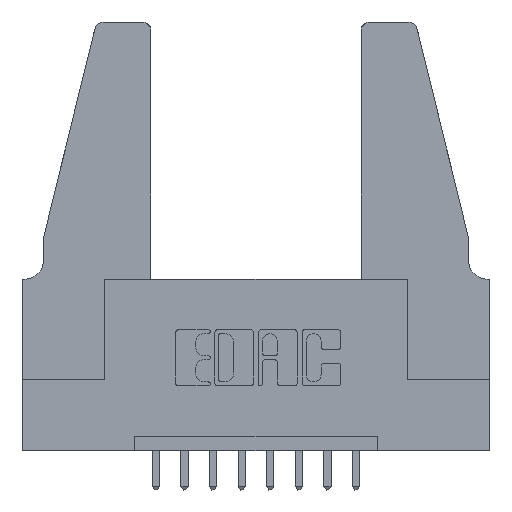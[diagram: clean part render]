
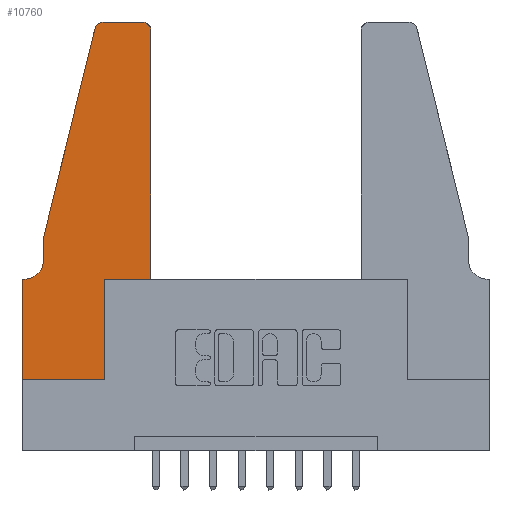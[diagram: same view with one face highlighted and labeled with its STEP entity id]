
A CAD part, top view. The second image highlights one B-rep face of the part: STEP entity #10760.
In plain terms, the highlighted planar face has unit normal (0, 0, 1).
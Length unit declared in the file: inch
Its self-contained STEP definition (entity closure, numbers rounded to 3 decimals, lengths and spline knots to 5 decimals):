
#9 = CARTESIAN_POINT ( 'NONE',  ( 0., 0.35, 0.37 ) ) ;
#29 = AXIS2_PLACEMENT_3D ( 'NONE', #9, #6821, #977 ) ;
#51 = ORIENTED_EDGE ( 'NONE', *, *, #4607, .T. ) ;
#342 = ORIENTED_EDGE ( 'NONE', *, *, #5918, .T. ) ;
#507 = VERTEX_POINT ( 'NONE', #11353 ) ;
#553 = DIRECTION ( 'NONE',  ( 0., -1., 0. ) ) ;
#571 = VECTOR ( 'NONE', #3005, 39.37008 ) ;
#877 = LINE ( 'NONE', #9490, #2388 ) ;
#940 = ORIENTED_EDGE ( 'NONE', *, *, #4984, .T. ) ;
#977 = DIRECTION ( 'NONE',  ( 1., 0., 0. ) ) ;
#985 = DIRECTION ( 'NONE',  ( -1., 0., 0. ) ) ;
#1038 = LINE ( 'NONE', #6354, #9707 ) ;
#1223 = VERTEX_POINT ( 'NONE', #7634 ) ;
#1245 = VERTEX_POINT ( 'NONE', #7879 ) ;
#1325 = VERTEX_POINT ( 'NONE', #9859 ) ;
#1500 = CARTESIAN_POINT ( 'NONE',  ( 0., 0.35, 0.37 ) ) ;
#1552 = CARTESIAN_POINT ( 'NONE',  ( 0., 0., 0.37 ) ) ;
#1948 = DIRECTION ( 'NONE',  ( 0., 0., 1. ) ) ;
#2105 = CARTESIAN_POINT ( 'NONE',  ( 0.0755, 0.5, 0.37 ) ) ;
#2178 = EDGE_CURVE ( 'NONE', #4876, #12113, #877, .T. ) ;
#2276 = LINE ( 'NONE', #6950, #5089 ) ;
#2388 = VECTOR ( 'NONE', #6645, 39.37008 ) ;
#2587 = CARTESIAN_POINT ( 'NONE',  ( 0.0755, 0.5, 0.37 ) ) ;
#2669 = ORIENTED_EDGE ( 'NONE', *, *, #11542, .T. ) ;
#3005 = DIRECTION ( 'NONE',  ( 0., 1., 0. ) ) ;
#3397 = CARTESIAN_POINT ( 'NONE',  ( 0.2865, 0., 0.37 ) ) ;
#3514 = EDGE_CURVE ( 'NONE', #1325, #11162, #4635, .T. ) ;
#3616 = CARTESIAN_POINT ( 'NONE',  ( 0.25487, 1.22718, 0.37 ) ) ;
#3918 = CARTESIAN_POINT ( 'NONE',  ( 0.4505, 0.35, 0.37 ) ) ;
#4117 = ORIENTED_EDGE ( 'NONE', *, *, #11129, .T. ) ;
#4183 = CARTESIAN_POINT ( 'NONE',  ( 0.0755, 0.42, 0.37 ) ) ;
#4236 = DIRECTION ( 'NONE',  ( -1., 0., 0. ) ) ;
#4283 = VECTOR ( 'NONE', #4236, 39.37008 ) ;
#4607 = EDGE_CURVE ( 'NONE', #7946, #507, #10639, .T. ) ;
#4635 = LINE ( 'NONE', #1552, #12669 ) ;
#4818 = PLANE ( 'NONE',  #29 ) ;
#4876 = VERTEX_POINT ( 'NONE', #3918 ) ;
#4931 = DIRECTION ( 'NONE',  ( 1., 0., 0. ) ) ;
#4984 = EDGE_CURVE ( 'NONE', #6380, #4876, #1038, .T. ) ;
#5089 = VECTOR ( 'NONE', #9927, 39.37008 ) ;
#5247 = VERTEX_POINT ( 'NONE', #2105 ) ;
#5677 = DIRECTION ( 'NONE',  ( 1., 0., 0. ) ) ;
#5882 = AXIS2_PLACEMENT_3D ( 'NONE', #9718, #9678, #12691 ) ;
#5918 = EDGE_CURVE ( 'NONE', #1245, #12586, #12764, .T. ) ;
#5923 = CARTESIAN_POINT ( 'NONE',  ( 0.0055, 0.42, 0.37 ) ) ;
#6045 = CARTESIAN_POINT ( 'NONE',  ( 0.2865, 0.35, 0.37 ) ) ;
#6167 = VECTOR ( 'NONE', #553, 39.37008 ) ;
#6354 = CARTESIAN_POINT ( 'NONE',  ( 0.4505, 0.35, 0.37 ) ) ;
#6380 = VERTEX_POINT ( 'NONE', #6488 ) ;
#6448 = AXIS2_PLACEMENT_3D ( 'NONE', #5923, #6925, #985 ) ;
#6488 = CARTESIAN_POINT ( 'NONE',  ( 0.2865, 0.35, 0.37 ) ) ;
#6645 = DIRECTION ( 'NONE',  ( 0., 1., 0. ) ) ;
#6821 = DIRECTION ( 'NONE',  ( 0., 0., 1. ) ) ;
#6925 = DIRECTION ( 'NONE',  ( 0., 0., -1. ) ) ;
#6950 = CARTESIAN_POINT ( 'NONE',  ( 0.0755, 0.35, 0.37 ) ) ;
#7523 = ORIENTED_EDGE ( 'NONE', *, *, #9766, .T. ) ;
#7634 = CARTESIAN_POINT ( 'NONE',  ( 0.4205, 1.25, 0.37 ) ) ;
#7635 = ORIENTED_EDGE ( 'NONE', *, *, #3514, .T. ) ;
#7644 = EDGE_LOOP ( 'NONE', ( #2669, #342, #12574, #8592, #51, #10507, #4117, #7635, #7523, #940, #10047, #9013 ) ) ;
#7724 = LINE ( 'NONE', #12223, #12016 ) ;
#7848 = LINE ( 'NONE', #9208, #4283 ) ;
#7879 = CARTESIAN_POINT ( 'NONE',  ( 0.284, 1.25, 0.37 ) ) ;
#7922 = CARTESIAN_POINT ( 'NONE',  ( 0.4505, 1.22, 0.37 ) ) ;
#7926 = VECTOR ( 'NONE', #11912, 39.37008 ) ;
#7946 = VERTEX_POINT ( 'NONE', #4183 ) ;
#8294 = DIRECTION ( 'NONE',  ( 0., -1., 0. ) ) ;
#8571 = EDGE_CURVE ( 'NONE', #12586, #5247, #12215, .T. ) ;
#8592 = ORIENTED_EDGE ( 'NONE', *, *, #10491, .T. ) ;
#9009 = CARTESIAN_POINT ( 'NONE',  ( 0.4205, 1.22, 0.37 ) ) ;
#9013 = ORIENTED_EDGE ( 'NONE', *, *, #11661, .T. ) ;
#9208 = CARTESIAN_POINT ( 'NONE',  ( 0.2605, 1.25, 0.37 ) ) ;
#9490 = CARTESIAN_POINT ( 'NONE',  ( 0.4505, 0.35, 0.37 ) ) ;
#9678 = DIRECTION ( 'NONE',  ( 0., 0., 1. ) ) ;
#9707 = VECTOR ( 'NONE', #11383, 39.37008 ) ;
#9718 = CARTESIAN_POINT ( 'NONE',  ( 0.284, 1.22, 0.37 ) ) ;
#9766 = EDGE_CURVE ( 'NONE', #11162, #6380, #10155, .T. ) ;
#9859 = CARTESIAN_POINT ( 'NONE',  ( 0., 0., 0.37 ) ) ;
#9927 = DIRECTION ( 'NONE',  ( -1., 0., 0. ) ) ;
#10047 = ORIENTED_EDGE ( 'NONE', *, *, #2178, .T. ) ;
#10109 = AXIS2_PLACEMENT_3D ( 'NONE', #9009, #1948, #4931 ) ;
#10155 = LINE ( 'NONE', #6045, #571 ) ;
#10390 = CARTESIAN_POINT ( 'NONE',  ( 0.0755, 0.5, 0.37 ) ) ;
#10491 = EDGE_CURVE ( 'NONE', #5247, #7946, #11578, .T. ) ;
#10507 = ORIENTED_EDGE ( 'NONE', *, *, #10699, .T. ) ;
#10639 = CIRCLE ( 'NONE', #6448, 0.07 ) ;
#10699 = EDGE_CURVE ( 'NONE', #507, #12460, #2276, .T. ) ;
#10760 = ADVANCED_FACE ( 'NONE', ( #11737 ), #4818, .T. ) ;
#11129 = EDGE_CURVE ( 'NONE', #12460, #1325, #7724, .T. ) ;
#11162 = VERTEX_POINT ( 'NONE', #3397 ) ;
#11353 = CARTESIAN_POINT ( 'NONE',  ( 0.0055, 0.35, 0.37 ) ) ;
#11383 = DIRECTION ( 'NONE',  ( 1., 0., 0. ) ) ;
#11542 = EDGE_CURVE ( 'NONE', #1223, #1245, #7848, .T. ) ;
#11578 = LINE ( 'NONE', #10390, #6167 ) ;
#11661 = EDGE_CURVE ( 'NONE', #12113, #1223, #12468, .T. ) ;
#11737 = FACE_OUTER_BOUND ( 'NONE', #7644, .T. ) ;
#11912 = DIRECTION ( 'NONE',  ( -0.239, -0.971, 0. ) ) ;
#12016 = VECTOR ( 'NONE', #8294, 39.37008 ) ;
#12113 = VERTEX_POINT ( 'NONE', #7922 ) ;
#12215 = LINE ( 'NONE', #2587, #7926 ) ;
#12223 = CARTESIAN_POINT ( 'NONE',  ( 0., 0., 0.37 ) ) ;
#12460 = VERTEX_POINT ( 'NONE', #1500 ) ;
#12468 = CIRCLE ( 'NONE', #10109, 0.03 ) ;
#12574 = ORIENTED_EDGE ( 'NONE', *, *, #8571, .T. ) ;
#12586 = VERTEX_POINT ( 'NONE', #3616 ) ;
#12669 = VECTOR ( 'NONE', #5677, 39.37008 ) ;
#12691 = DIRECTION ( 'NONE',  ( 1., 0., 0. ) ) ;
#12764 = CIRCLE ( 'NONE', #5882, 0.03 ) ;
